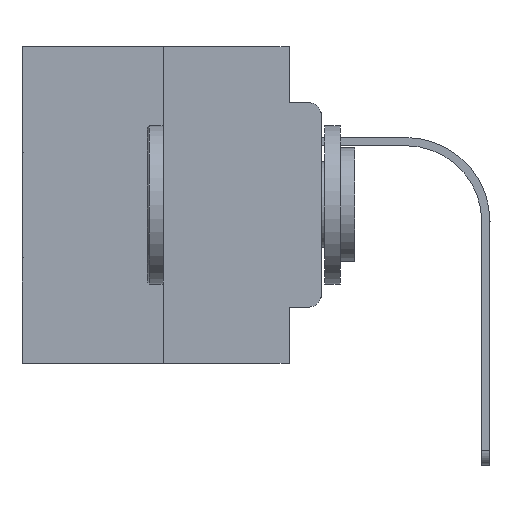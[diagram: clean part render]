
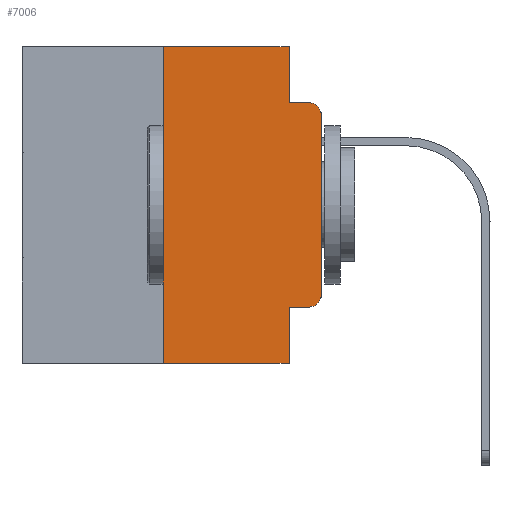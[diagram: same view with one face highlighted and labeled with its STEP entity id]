
A CAD part, left-side view. The second image highlights one B-rep face of the part: STEP entity #7006.
In plain terms, the highlighted planar face has unit normal (-1, 0, 0).
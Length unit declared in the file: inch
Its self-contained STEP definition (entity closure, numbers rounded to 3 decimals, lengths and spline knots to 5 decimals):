
#607 = LINE ( 'NONE', #16173, #21904 ) ;
#1140 = ORIENTED_EDGE ( 'NONE', *, *, #11226, .T. ) ;
#1207 = CARTESIAN_POINT ( 'NONE',  ( 0., 0., -0.1085 ) ) ;
#1274 = CIRCLE ( 'NONE', #19597, 0.02 ) ;
#1317 = VECTOR ( 'NONE', #14925, 39.37008 ) ;
#1661 = EDGE_CURVE ( 'NONE', #11565, #21395, #1274, .T. ) ;
#2308 = VECTOR ( 'NONE', #23668, 39.37008 ) ;
#3270 = ORIENTED_EDGE ( 'NONE', *, *, #13871, .T. ) ;
#3322 = ORIENTED_EDGE ( 'NONE', *, *, #19652, .T. ) ;
#3791 = EDGE_CURVE ( 'NONE', #23005, #20548, #607, .T. ) ;
#3956 = DIRECTION ( 'NONE',  ( 0., -1., 0. ) ) ;
#5707 = CARTESIAN_POINT ( 'NONE',  ( 0., 0.25, 0. ) ) ;
#6087 = CARTESIAN_POINT ( 'NONE',  ( 0., 0.051, -0.5 ) ) ;
#6287 = CARTESIAN_POINT ( 'NONE',  ( 0., 0.051, -0.0885 ) ) ;
#6587 = DIRECTION ( 'NONE',  ( 0., -1., 0. ) ) ;
#6588 = VECTOR ( 'NONE', #17758, 39.37008 ) ;
#7006 = ADVANCED_FACE ( 'NONE', ( #7852 ), #17423, .F. ) ;
#7852 = FACE_OUTER_BOUND ( 'NONE', #22700, .T. ) ;
#7946 = VERTEX_POINT ( 'NONE', #12609 ) ;
#9232 = VERTEX_POINT ( 'NONE', #24730 ) ;
#9736 = VECTOR ( 'NONE', #28240, 39.37008 ) ;
#10327 = ORIENTED_EDGE ( 'NONE', *, *, #15994, .F. ) ;
#10369 = CARTESIAN_POINT ( 'NONE',  ( 0., 0., 0. ) ) ;
#10706 = CARTESIAN_POINT ( 'NONE',  ( 0., 0.473, 0. ) ) ;
#11226 = EDGE_CURVE ( 'NONE', #22319, #16040, #18610, .T. ) ;
#11565 = VERTEX_POINT ( 'NONE', #1207 ) ;
#12117 = DIRECTION ( 'NONE',  ( 0., 0., -1. ) ) ;
#12461 = CARTESIAN_POINT ( 'NONE',  ( 0., 0.02, -0.3915 ) ) ;
#12609 = CARTESIAN_POINT ( 'NONE',  ( 0., 0.25, -0.5 ) ) ;
#12856 = CARTESIAN_POINT ( 'NONE',  ( 0., 0.473, 0. ) ) ;
#13371 = CARTESIAN_POINT ( 'NONE',  ( 0., 0., -0.3915 ) ) ;
#13857 = EDGE_CURVE ( 'NONE', #20548, #21395, #15132, .T. ) ;
#13871 = EDGE_CURVE ( 'NONE', #7946, #16062, #24265, .T. ) ;
#14925 = DIRECTION ( 'NONE',  ( 0., 0., 1. ) ) ;
#15132 = LINE ( 'NONE', #6287, #28735 ) ;
#15143 = ORIENTED_EDGE ( 'NONE', *, *, #1661, .T. ) ;
#15994 = EDGE_CURVE ( 'NONE', #22319, #16062, #17275, .T. ) ;
#16040 = VERTEX_POINT ( 'NONE', #26016 ) ;
#16062 = VERTEX_POINT ( 'NONE', #6087 ) ;
#16173 = CARTESIAN_POINT ( 'NONE',  ( 0., 0.051, 0. ) ) ;
#16228 = CIRCLE ( 'NONE', #22820, 0.02 ) ;
#16323 = DIRECTION ( 'NONE',  ( 0., 0., -1. ) ) ;
#17003 = ORIENTED_EDGE ( 'NONE', *, *, #28144, .T. ) ;
#17084 = CARTESIAN_POINT ( 'NONE',  ( 0., 0.051, -0.4115 ) ) ;
#17275 = LINE ( 'NONE', #23914, #22621 ) ;
#17423 = PLANE ( 'NONE',  #28656 ) ;
#17758 = DIRECTION ( 'NONE',  ( 0., -1., 0. ) ) ;
#18577 = DIRECTION ( 'NONE',  ( -1., 0., 0. ) ) ;
#18610 = LINE ( 'NONE', #25884, #9736 ) ;
#19597 = AXIS2_PLACEMENT_3D ( 'NONE', #27464, #18577, #12117 ) ;
#19652 = EDGE_CURVE ( 'NONE', #16040, #22607, #16228, .T. ) ;
#20287 = ORIENTED_EDGE ( 'NONE', *, *, #27804, .F. ) ;
#20389 = CARTESIAN_POINT ( 'NONE',  ( 0., 0.051, 0. ) ) ;
#20548 = VERTEX_POINT ( 'NONE', #26549 ) ;
#20802 = ORIENTED_EDGE ( 'NONE', *, *, #3791, .F. ) ;
#21395 = VERTEX_POINT ( 'NONE', #22505 ) ;
#21428 = DIRECTION ( 'NONE',  ( -1., 0., 0. ) ) ;
#21882 = CARTESIAN_POINT ( 'NONE',  ( 0., 0.473, -0.5 ) ) ;
#21903 = ORIENTED_EDGE ( 'NONE', *, *, #13857, .F. ) ;
#21904 = VECTOR ( 'NONE', #16323, 39.37008 ) ;
#22319 = VERTEX_POINT ( 'NONE', #17084 ) ;
#22505 = CARTESIAN_POINT ( 'NONE',  ( 0., 0.02, -0.0885 ) ) ;
#22607 = VERTEX_POINT ( 'NONE', #13371 ) ;
#22621 = VECTOR ( 'NONE', #26567, 39.37008 ) ;
#22700 = EDGE_LOOP ( 'NONE', ( #17003, #15143, #21903, #20802, #28880, #20287, #3270, #10327, #1140, #3322 ) ) ;
#22820 = AXIS2_PLACEMENT_3D ( 'NONE', #12461, #21428, #25467 ) ;
#23005 = VERTEX_POINT ( 'NONE', #20389 ) ;
#23668 = DIRECTION ( 'NONE',  ( 0., 0., 1. ) ) ;
#23914 = CARTESIAN_POINT ( 'NONE',  ( 0., 0.051, 0. ) ) ;
#24117 = EDGE_CURVE ( 'NONE', #9232, #23005, #28849, .T. ) ;
#24265 = LINE ( 'NONE', #21882, #6588 ) ;
#24730 = CARTESIAN_POINT ( 'NONE',  ( 0., 0.25, 0. ) ) ;
#25467 = DIRECTION ( 'NONE',  ( 0., 0., -1. ) ) ;
#25865 = LINE ( 'NONE', #10369, #1317 ) ;
#25884 = CARTESIAN_POINT ( 'NONE',  ( 0., 0.051, -0.4115 ) ) ;
#25901 = LINE ( 'NONE', #5707, #2308 ) ;
#26016 = CARTESIAN_POINT ( 'NONE',  ( 0., 0.02, -0.4115 ) ) ;
#26549 = CARTESIAN_POINT ( 'NONE',  ( 0., 0.051, -0.0885 ) ) ;
#26567 = DIRECTION ( 'NONE',  ( 0., 0., -1. ) ) ;
#27016 = VECTOR ( 'NONE', #6587, 39.37008 ) ;
#27464 = CARTESIAN_POINT ( 'NONE',  ( 0., 0.02, -0.1085 ) ) ;
#27804 = EDGE_CURVE ( 'NONE', #7946, #9232, #25901, .T. ) ;
#28144 = EDGE_CURVE ( 'NONE', #22607, #11565, #25865, .T. ) ;
#28240 = DIRECTION ( 'NONE',  ( 0., -1., 0. ) ) ;
#28369 = DIRECTION ( 'NONE',  ( 1., 0., 0. ) ) ;
#28651 = DIRECTION ( 'NONE',  ( 0., 0., -1. ) ) ;
#28656 = AXIS2_PLACEMENT_3D ( 'NONE', #12856, #28369, #28651 ) ;
#28735 = VECTOR ( 'NONE', #3956, 39.37008 ) ;
#28849 = LINE ( 'NONE', #10706, #27016 ) ;
#28880 = ORIENTED_EDGE ( 'NONE', *, *, #24117, .F. ) ;
